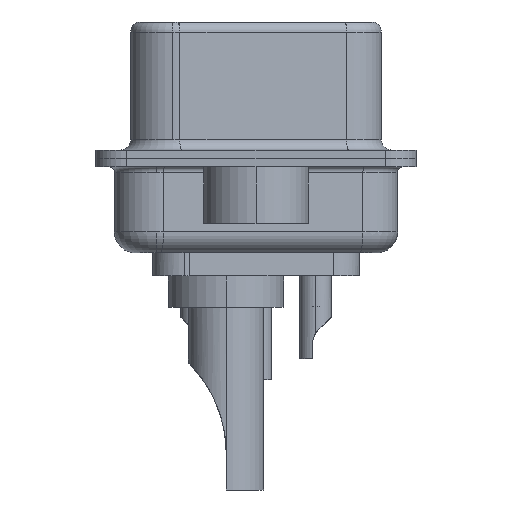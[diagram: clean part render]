
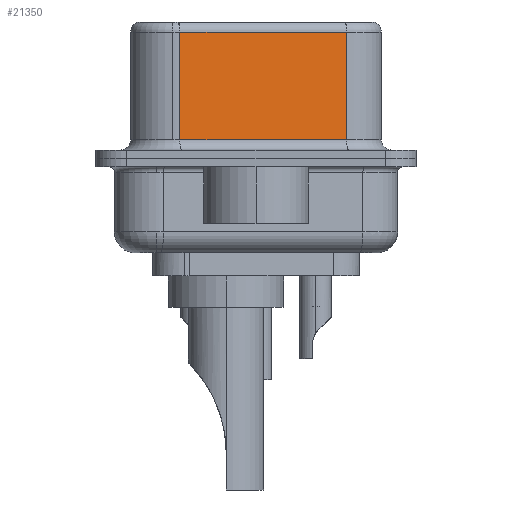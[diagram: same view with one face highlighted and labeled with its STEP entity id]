
A CAD part, left-side view. The second image highlights one B-rep face of the part: STEP entity #21350.
In plain terms, the highlighted planar face has unit normal (-0.985, -0.174, 0).
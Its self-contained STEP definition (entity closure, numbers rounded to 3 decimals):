
#29 = CARTESIAN_POINT ( 'NONE',  ( 5.132, -4.322, 6.02 ) ) ;
#1010 = CARTESIAN_POINT ( 'NONE',  ( 5.132, -4.322, 6.52 ) ) ;
#2420 = CARTESIAN_POINT ( 'NONE',  ( 5.132, -4.322, 6.52 ) ) ;
#3151 = DIRECTION ( 'NONE',  ( 0.985, 0.174, 0. ) ) ;
#3402 = VERTEX_POINT ( 'NONE', #14029 ) ;
#3466 = CARTESIAN_POINT ( 'NONE',  ( 5.132, -4.322, 0.9 ) ) ;
#3469 = ORIENTED_EDGE ( 'NONE', *, *, #21135, .F. ) ;
#4109 = VECTOR ( 'NONE', #10417, 1000. ) ;
#4489 = DIRECTION ( 'NONE',  ( 0., 0., -1. ) ) ;
#4836 = VECTOR ( 'NONE', #11444, 1000. ) ;
#5576 = EDGE_CURVE ( 'NONE', #8698, #20262, #11141, .T. ) ;
#7988 = EDGE_LOOP ( 'NONE', ( #3469, #8316, #8290, #23292 ) ) ;
#8290 = ORIENTED_EDGE ( 'NONE', *, *, #15995, .T. ) ;
#8316 = ORIENTED_EDGE ( 'NONE', *, *, #22807, .T. ) ;
#8698 = VERTEX_POINT ( 'NONE', #15651 ) ;
#9185 = LINE ( 'NONE', #2420, #24732 ) ;
#9301 = AXIS2_PLACEMENT_3D ( 'NONE', #1010, #3151, #17584 ) ;
#9784 = VERTEX_POINT ( 'NONE', #29 ) ;
#9921 = VECTOR ( 'NONE', #19337, 1000. ) ;
#10417 = DIRECTION ( 'NONE',  ( -0.174, 0.985, 0. ) ) ;
#10554 = LINE ( 'NONE', #25484, #9921 ) ;
#11141 = LINE ( 'NONE', #25614, #4836 ) ;
#11444 = DIRECTION ( 'NONE',  ( 0.174, -0.985, 0. ) ) ;
#13557 = PLANE ( 'NONE',  #9301 ) ;
#14029 = CARTESIAN_POINT ( 'NONE',  ( 3.73, 3.628, 6.02 ) ) ;
#15651 = CARTESIAN_POINT ( 'NONE',  ( 3.73, 3.628, 0.9 ) ) ;
#15995 = EDGE_CURVE ( 'NONE', #3402, #8698, #10554, .T. ) ;
#17584 = DIRECTION ( 'NONE',  ( -0.174, 0.985, 0. ) ) ;
#19337 = DIRECTION ( 'NONE',  ( 0., 0., -1. ) ) ;
#19898 = LINE ( 'NONE', #22551, #4109 ) ;
#20262 = VERTEX_POINT ( 'NONE', #3466 ) ;
#20289 = FACE_OUTER_BOUND ( 'NONE', #7988, .T. ) ;
#21135 = EDGE_CURVE ( 'NONE', #9784, #20262, #9185, .T. ) ;
#21350 = ADVANCED_FACE ( 'NONE', ( #20289 ), #13557, .F. ) ;
#22551 = CARTESIAN_POINT ( 'NONE',  ( 5.132, -4.322, 6.02 ) ) ;
#22807 = EDGE_CURVE ( 'NONE', #9784, #3402, #19898, .T. ) ;
#23292 = ORIENTED_EDGE ( 'NONE', *, *, #5576, .T. ) ;
#24732 = VECTOR ( 'NONE', #4489, 1000. ) ;
#25484 = CARTESIAN_POINT ( 'NONE',  ( 3.73, 3.628, 6.52 ) ) ;
#25614 = CARTESIAN_POINT ( 'NONE',  ( 5.132, -4.322, 0.9 ) ) ;
